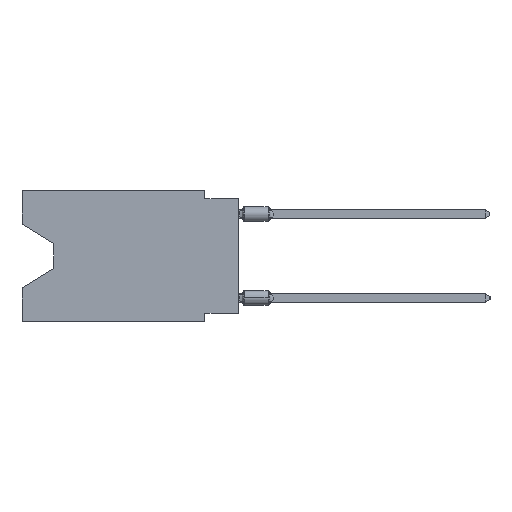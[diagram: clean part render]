
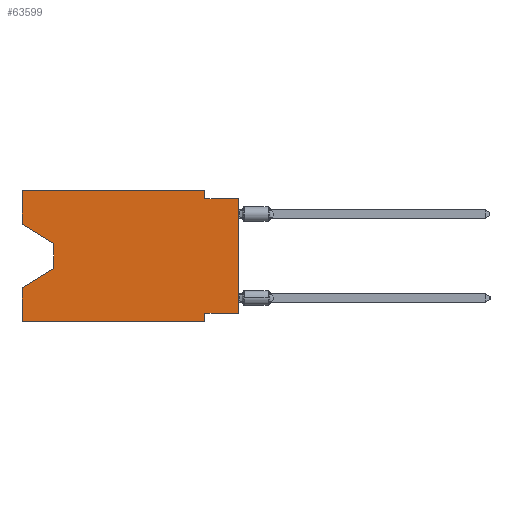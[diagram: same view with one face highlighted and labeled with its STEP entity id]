
A CAD part, left-side view. The second image highlights one B-rep face of the part: STEP entity #63599.
In plain terms, the highlighted planar face has unit normal (-1, 0, 0).
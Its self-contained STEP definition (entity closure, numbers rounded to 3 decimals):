
#1254 = EDGE_CURVE ( 'NONE', #19538, #14697, #14650, .T. ) ;
#1579 = VERTEX_POINT ( 'NONE', #57265 ) ;
#1694 = EDGE_CURVE ( 'NONE', #39453, #13477, #5077, .T. ) ;
#3127 = ORIENTED_EDGE ( 'NONE', *, *, #62806, .F. ) ;
#3524 = ORIENTED_EDGE ( 'NONE', *, *, #11998, .T. ) ;
#4994 = EDGE_CURVE ( 'NONE', #39453, #14697, #62179, .T. ) ;
#5077 = LINE ( 'NONE', #24084, #34414 ) ;
#5508 = EDGE_CURVE ( 'NONE', #31207, #45457, #34089, .T. ) ;
#5577 = CARTESIAN_POINT ( 'NONE',  ( 0., 13.97, -4.013 ) ) ;
#6592 = DIRECTION ( 'NONE',  ( 0., 0., 1. ) ) ;
#7006 = ORIENTED_EDGE ( 'NONE', *, *, #25498, .F. ) ;
#7017 = VECTOR ( 'NONE', #38807, 1000. ) ;
#7108 = EDGE_CURVE ( 'NONE', #45457, #13477, #38709, .T. ) ;
#8373 = VECTOR ( 'NONE', #51010, 1000. ) ;
#8501 = DIRECTION ( 'NONE',  ( 0., 0., -1. ) ) ;
#10164 = CARTESIAN_POINT ( 'NONE',  ( 0., 2.54, -9.906 ) ) ;
#10891 = EDGE_CURVE ( 'NONE', #38639, #31207, #40236, .T. ) ;
#11025 = VECTOR ( 'NONE', #31692, 1000. ) ;
#11867 = VECTOR ( 'NONE', #61799, 1000. ) ;
#11998 = EDGE_CURVE ( 'NONE', #31776, #61327, #16090, .T. ) ;
#13477 = VERTEX_POINT ( 'NONE', #39976 ) ;
#14304 = VECTOR ( 'NONE', #6592, 1000. ) ;
#14380 = PLANE ( 'NONE',  #32866 ) ;
#14650 = LINE ( 'NONE', #59591, #17618 ) ;
#14697 = VERTEX_POINT ( 'NONE', #10164 ) ;
#16090 = LINE ( 'NONE', #41313, #14304 ) ;
#17618 = VECTOR ( 'NONE', #29397, 1000. ) ;
#18309 = CARTESIAN_POINT ( 'NONE',  ( 0., 13.97, -5.893 ) ) ;
#18332 = CARTESIAN_POINT ( 'NONE',  ( 0., 16.383, 0. ) ) ;
#18436 = CARTESIAN_POINT ( 'NONE',  ( 0., 16.383, 0. ) ) ;
#19538 = VERTEX_POINT ( 'NONE', #43539 ) ;
#21046 = ORIENTED_EDGE ( 'NONE', *, *, #5508, .T. ) ;
#21144 = LINE ( 'NONE', #60200, #8373 ) ;
#21785 = LINE ( 'NONE', #37494, #11867 ) ;
#21825 = VECTOR ( 'NONE', #23350, 1000. ) ;
#22235 = VECTOR ( 'NONE', #53831, 1000. ) ;
#23350 = DIRECTION ( 'NONE',  ( 0., -1., 0. ) ) ;
#23678 = ORIENTED_EDGE ( 'NONE', *, *, #1254, .F. ) ;
#24084 = CARTESIAN_POINT ( 'NONE',  ( 0., 16.383, 0. ) ) ;
#25498 = EDGE_CURVE ( 'NONE', #31776, #19538, #64729, .T. ) ;
#25563 = DIRECTION ( 'NONE',  ( 0., 0., -1. ) ) ;
#29397 = DIRECTION ( 'NONE',  ( 0., 0., -1. ) ) ;
#31207 = VERTEX_POINT ( 'NONE', #41483 ) ;
#31430 = EDGE_CURVE ( 'NONE', #47305, #61327, #62377, .T. ) ;
#31692 = DIRECTION ( 'NONE',  ( 0., -0.855, -0.519 ) ) ;
#31776 = VERTEX_POINT ( 'NONE', #56232 ) ;
#31912 = CARTESIAN_POINT ( 'NONE',  ( 0., 16.383, 0. ) ) ;
#32124 = ORIENTED_EDGE ( 'NONE', *, *, #7108, .T. ) ;
#32866 = AXIS2_PLACEMENT_3D ( 'NONE', #18332, #64238, #8501 ) ;
#33149 = CARTESIAN_POINT ( 'NONE',  ( 0., 13.97, -5.893 ) ) ;
#33804 = CARTESIAN_POINT ( 'NONE',  ( 0., 16.383, -9.906 ) ) ;
#34089 = LINE ( 'NONE', #5577, #45137 ) ;
#34414 = VECTOR ( 'NONE', #64111, 1000. ) ;
#34537 = CARTESIAN_POINT ( 'NONE',  ( 0., 0., -9.271 ) ) ;
#36120 = DIRECTION ( 'NONE',  ( 0., -1., 0. ) ) ;
#37433 = EDGE_CURVE ( 'NONE', #1579, #47305, #21144, .T. ) ;
#37494 = CARTESIAN_POINT ( 'NONE',  ( 0., 16.383, 0. ) ) ;
#37674 = ORIENTED_EDGE ( 'NONE', *, *, #37433, .F. ) ;
#38639 = VERTEX_POINT ( 'NONE', #59891 ) ;
#38709 = LINE ( 'NONE', #33149, #22235 ) ;
#38807 = DIRECTION ( 'NONE',  ( 0., 1., 0. ) ) ;
#39418 = ORIENTED_EDGE ( 'NONE', *, *, #4994, .T. ) ;
#39453 = VERTEX_POINT ( 'NONE', #33804 ) ;
#39844 = CARTESIAN_POINT ( 'NONE',  ( 0., 2.54, -0.635 ) ) ;
#39976 = CARTESIAN_POINT ( 'NONE',  ( 0., 16.383, -7.36 ) ) ;
#40236 = LINE ( 'NONE', #51079, #11025 ) ;
#40391 = VERTEX_POINT ( 'NONE', #31912 ) ;
#40951 = ORIENTED_EDGE ( 'NONE', *, *, #10891, .T. ) ;
#41313 = CARTESIAN_POINT ( 'NONE',  ( 0., 0., 0. ) ) ;
#41483 = CARTESIAN_POINT ( 'NONE',  ( 0., 13.97, -4.013 ) ) ;
#42430 = VECTOR ( 'NONE', #36120, 1000. ) ;
#42939 = VECTOR ( 'NONE', #64123, 1000. ) ;
#43539 = CARTESIAN_POINT ( 'NONE',  ( 0., 2.54, -9.271 ) ) ;
#43673 = LINE ( 'NONE', #18436, #21825 ) ;
#44417 = CARTESIAN_POINT ( 'NONE',  ( 0., 16.383, -9.906 ) ) ;
#45088 = ORIENTED_EDGE ( 'NONE', *, *, #31430, .F. ) ;
#45137 = VECTOR ( 'NONE', #25563, 1000. ) ;
#45457 = VERTEX_POINT ( 'NONE', #18309 ) ;
#47305 = VERTEX_POINT ( 'NONE', #39844 ) ;
#51010 = DIRECTION ( 'NONE',  ( 0., 0., -1. ) ) ;
#51079 = CARTESIAN_POINT ( 'NONE',  ( 0., 16.383, -2.546 ) ) ;
#51442 = EDGE_CURVE ( 'NONE', #40391, #1579, #43673, .T. ) ;
#52203 = CARTESIAN_POINT ( 'NONE',  ( 0., 0., -0.635 ) ) ;
#53831 = DIRECTION ( 'NONE',  ( 0., 0.855, -0.519 ) ) ;
#55792 = ORIENTED_EDGE ( 'NONE', *, *, #1694, .F. ) ;
#56232 = CARTESIAN_POINT ( 'NONE',  ( 0., 0., -9.271 ) ) ;
#57265 = CARTESIAN_POINT ( 'NONE',  ( 0., 2.54, 0. ) ) ;
#57604 = CARTESIAN_POINT ( 'NONE',  ( 0., 0., -0.635 ) ) ;
#58754 = EDGE_LOOP ( 'NONE', ( #40951, #21046, #32124, #55792, #39418, #23678, #7006, #3524, #45088, #37674, #63093, #3127 ) ) ;
#58985 = FACE_OUTER_BOUND ( 'NONE', #58754, .T. ) ;
#59591 = CARTESIAN_POINT ( 'NONE',  ( 0., 2.54, -9.906 ) ) ;
#59891 = CARTESIAN_POINT ( 'NONE',  ( 0., 16.383, -2.546 ) ) ;
#60200 = CARTESIAN_POINT ( 'NONE',  ( 0., 2.54, 0. ) ) ;
#61327 = VERTEX_POINT ( 'NONE', #57604 ) ;
#61799 = DIRECTION ( 'NONE',  ( 0., 0., 1. ) ) ;
#62179 = LINE ( 'NONE', #44417, #42939 ) ;
#62377 = LINE ( 'NONE', #52203, #42430 ) ;
#62806 = EDGE_CURVE ( 'NONE', #38639, #40391, #21785, .T. ) ;
#63093 = ORIENTED_EDGE ( 'NONE', *, *, #51442, .F. ) ;
#63599 = ADVANCED_FACE ( 'NONE', ( #58985 ), #14380, .F. ) ;
#64111 = DIRECTION ( 'NONE',  ( 0., 0., 1. ) ) ;
#64123 = DIRECTION ( 'NONE',  ( 0., -1., 0. ) ) ;
#64238 = DIRECTION ( 'NONE',  ( 1., 0., 0. ) ) ;
#64729 = LINE ( 'NONE', #34537, #7017 ) ;
